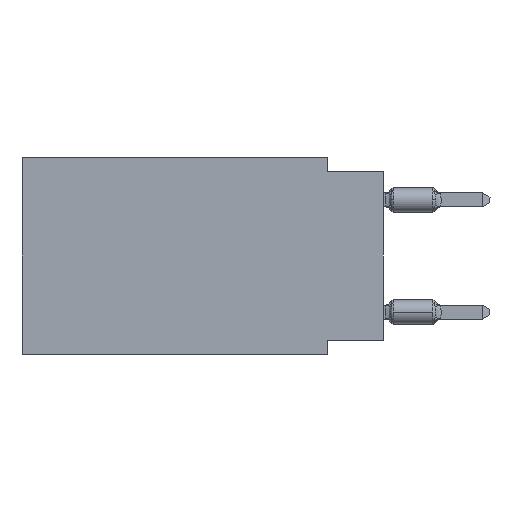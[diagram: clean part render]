
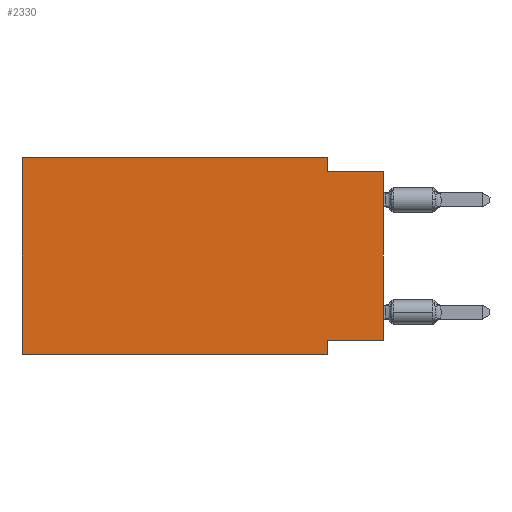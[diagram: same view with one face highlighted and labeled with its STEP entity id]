
A CAD part, left-side view. The second image highlights one B-rep face of the part: STEP entity #2330.
In plain terms, the highlighted planar face has unit normal (-1, 0, 0).
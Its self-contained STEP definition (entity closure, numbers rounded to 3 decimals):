
#156 = ORIENTED_EDGE ( 'NONE', *, *, #2798, .F. ) ;
#159 = CARTESIAN_POINT ( 'NONE',  ( 0., 16.383, 0. ) ) ;
#240 = CARTESIAN_POINT ( 'NONE',  ( 0., 0., -0.635 ) ) ;
#243 = VERTEX_POINT ( 'NONE', #11424 ) ;
#316 = LINE ( 'NONE', #1278, #7094 ) ;
#348 = DIRECTION ( 'NONE',  ( 0., 0., 1. ) ) ;
#935 = DIRECTION ( 'NONE',  ( 0., -1., 0. ) ) ;
#1045 = LINE ( 'NONE', #5269, #4615 ) ;
#1278 = CARTESIAN_POINT ( 'NONE',  ( 0., 0., -8.255 ) ) ;
#1345 = VECTOR ( 'NONE', #12887, 1000. ) ;
#1357 = VECTOR ( 'NONE', #3332, 1000. ) ;
#1467 = AXIS2_PLACEMENT_3D ( 'NONE', #6241, #2092, #11345 ) ;
#1477 = ORIENTED_EDGE ( 'NONE', *, *, #3499, .F. ) ;
#1483 = ORIENTED_EDGE ( 'NONE', *, *, #4438, .T. ) ;
#1614 = ORIENTED_EDGE ( 'NONE', *, *, #12665, .F. ) ;
#1966 = LINE ( 'NONE', #8450, #2685 ) ;
#1972 = EDGE_CURVE ( 'NONE', #5278, #3942, #7639, .T. ) ;
#2092 = DIRECTION ( 'NONE',  ( 1., 0., 0. ) ) ;
#2330 = ADVANCED_FACE ( 'NONE', ( #2940 ), #9221, .F. ) ;
#2524 = LINE ( 'NONE', #12045, #5787 ) ;
#2617 = CARTESIAN_POINT ( 'NONE',  ( 0., 0., -0.635 ) ) ;
#2685 = VECTOR ( 'NONE', #935, 1000. ) ;
#2798 = EDGE_CURVE ( 'NONE', #243, #4026, #1045, .T. ) ;
#2940 = FACE_OUTER_BOUND ( 'NONE', #11078, .T. ) ;
#3215 = VECTOR ( 'NONE', #11839, 1000. ) ;
#3332 = DIRECTION ( 'NONE',  ( 0., 0., 1. ) ) ;
#3499 = EDGE_CURVE ( 'NONE', #12554, #243, #1966, .T. ) ;
#3531 = VERTEX_POINT ( 'NONE', #240 ) ;
#3781 = CARTESIAN_POINT ( 'NONE',  ( 0., 2.54, -8.255 ) ) ;
#3942 = VERTEX_POINT ( 'NONE', #7603 ) ;
#4026 = VERTEX_POINT ( 'NONE', #5406 ) ;
#4438 = EDGE_CURVE ( 'NONE', #5569, #3531, #8763, .T. ) ;
#4615 = VECTOR ( 'NONE', #9467, 1000. ) ;
#4897 = CARTESIAN_POINT ( 'NONE',  ( 0., 0., -8.255 ) ) ;
#4996 = ORIENTED_EDGE ( 'NONE', *, *, #7287, .F. ) ;
#5269 = CARTESIAN_POINT ( 'NONE',  ( 0., 2.54, 0. ) ) ;
#5278 = VERTEX_POINT ( 'NONE', #11585 ) ;
#5406 = CARTESIAN_POINT ( 'NONE',  ( 0., 2.54, -0.635 ) ) ;
#5504 = CARTESIAN_POINT ( 'NONE',  ( 0., 16.383, -8.89 ) ) ;
#5569 = VERTEX_POINT ( 'NONE', #4897 ) ;
#5787 = VECTOR ( 'NONE', #7629, 1000. ) ;
#5862 = LINE ( 'NONE', #2617, #1345 ) ;
#6002 = ORIENTED_EDGE ( 'NONE', *, *, #12030, .F. ) ;
#6241 = CARTESIAN_POINT ( 'NONE',  ( 0., 16.383, 0. ) ) ;
#6669 = DIRECTION ( 'NONE',  ( 0., 1., 0. ) ) ;
#7094 = VECTOR ( 'NONE', #6669, 1000. ) ;
#7286 = EDGE_CURVE ( 'NONE', #12254, #3942, #2524, .T. ) ;
#7287 = EDGE_CURVE ( 'NONE', #5569, #12254, #316, .T. ) ;
#7603 = CARTESIAN_POINT ( 'NONE',  ( 0., 2.54, -8.89 ) ) ;
#7629 = DIRECTION ( 'NONE',  ( 0., 0., -1. ) ) ;
#7639 = LINE ( 'NONE', #5504, #3215 ) ;
#8450 = CARTESIAN_POINT ( 'NONE',  ( 0., 16.383, 0. ) ) ;
#8506 = LINE ( 'NONE', #159, #1357 ) ;
#8763 = LINE ( 'NONE', #10621, #13607 ) ;
#8780 = ORIENTED_EDGE ( 'NONE', *, *, #7286, .F. ) ;
#9221 = PLANE ( 'NONE',  #1467 ) ;
#9467 = DIRECTION ( 'NONE',  ( 0., 0., -1. ) ) ;
#10621 = CARTESIAN_POINT ( 'NONE',  ( 0., 0., 0. ) ) ;
#11078 = EDGE_LOOP ( 'NONE', ( #1483, #6002, #156, #1477, #1614, #12974, #8780, #4996 ) ) ;
#11345 = DIRECTION ( 'NONE',  ( 0., 0., -1. ) ) ;
#11424 = CARTESIAN_POINT ( 'NONE',  ( 0., 2.54, 0. ) ) ;
#11585 = CARTESIAN_POINT ( 'NONE',  ( 0., 16.383, -8.89 ) ) ;
#11835 = CARTESIAN_POINT ( 'NONE',  ( 0., 16.383, 0. ) ) ;
#11839 = DIRECTION ( 'NONE',  ( 0., -1., 0. ) ) ;
#12030 = EDGE_CURVE ( 'NONE', #4026, #3531, #5862, .T. ) ;
#12045 = CARTESIAN_POINT ( 'NONE',  ( 0., 2.54, -8.89 ) ) ;
#12254 = VERTEX_POINT ( 'NONE', #3781 ) ;
#12554 = VERTEX_POINT ( 'NONE', #11835 ) ;
#12665 = EDGE_CURVE ( 'NONE', #5278, #12554, #8506, .T. ) ;
#12887 = DIRECTION ( 'NONE',  ( 0., -1., 0. ) ) ;
#12974 = ORIENTED_EDGE ( 'NONE', *, *, #1972, .T. ) ;
#13607 = VECTOR ( 'NONE', #348, 1000. ) ;
